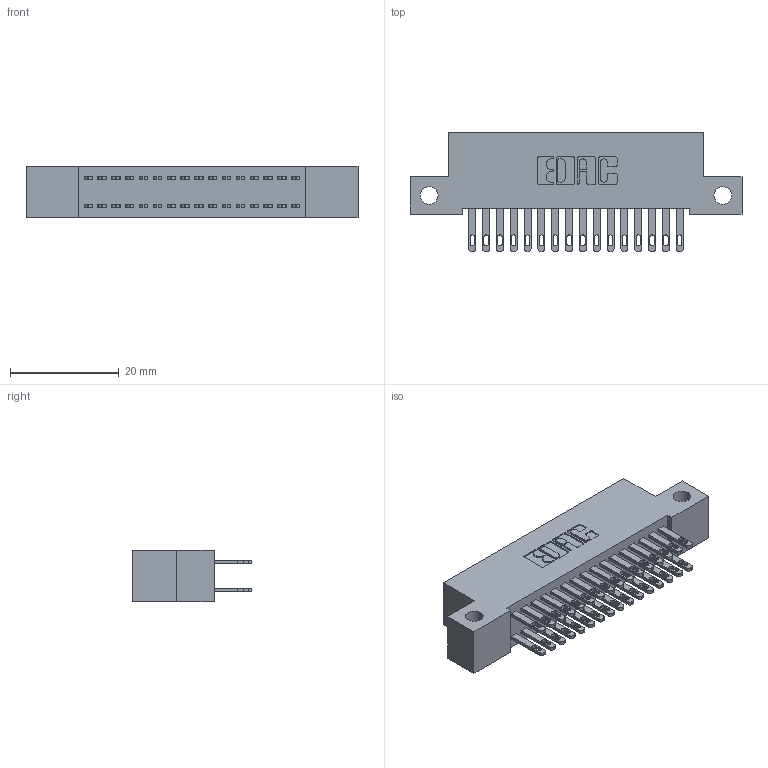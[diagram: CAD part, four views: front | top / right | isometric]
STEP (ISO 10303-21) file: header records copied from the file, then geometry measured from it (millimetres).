
FILE_DESCRIPTION (( 'STEP AP203' ), '1' );
FILE_NAME ('342-032-500-212.STEP', '2018-08-11T16:33:03', ( '' ), ( '' ), 'SwSTEP 2.0', 'SolidWorks 2016', '' );
FILE_SCHEMA (( 'CONFIG_CONTROL_DESIGN' ));
Length unit declared in the file: inch
Products named in the file (3): 342 Part_Side Mount; 345-292-001_345-293-100; 342-032-500-212
Assembly tree (33 placements, depth 2):
  342-032-500-212
    342 Part_Side Mount
    345-292-001_345-293-100  x32
Bounding box: 60.96 x 21.85 x 9.4 mm (x, y, z)
Volume: 5378 mm3; surface area: 8260.1 mm2
Topology: 33 solids, 33 shells, 1646 faces, 5003 edges, 3334 vertices
Faces by surface type: plane 1026, cylinder 620
Entity records: 13457 total; most frequent: CARTESIAN_POINT 2258, ORIENTED_EDGE 2194, DIRECTION 1977, EDGE_CURVE 1097, LINE 965, VECTOR 965, VERTEX_POINT 730, AXIS2_PLACEMENT_3D 506
